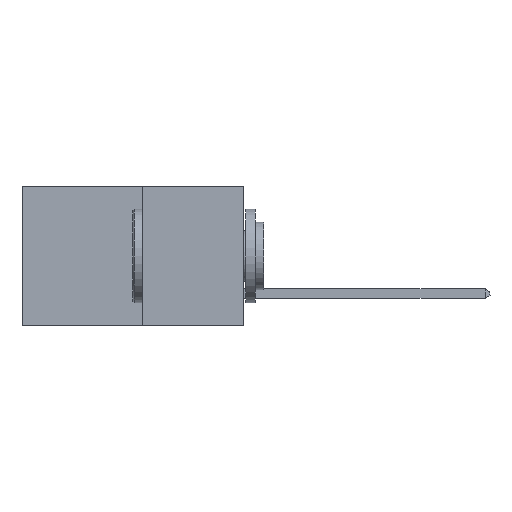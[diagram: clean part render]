
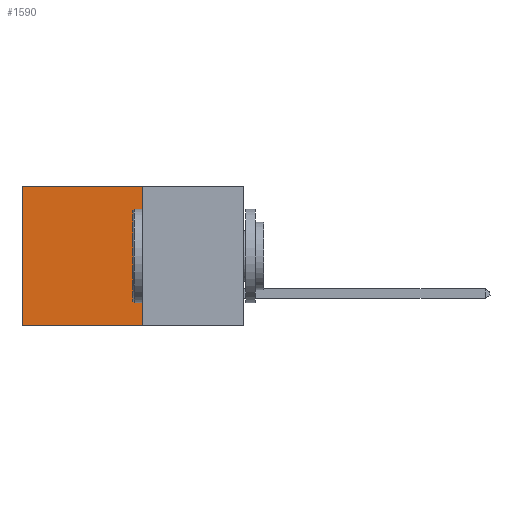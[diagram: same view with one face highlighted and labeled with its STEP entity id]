
A CAD part, left-side view. The second image highlights one B-rep face of the part: STEP entity #1590.
In plain terms, the highlighted planar face has unit normal (-1, 0, 0).
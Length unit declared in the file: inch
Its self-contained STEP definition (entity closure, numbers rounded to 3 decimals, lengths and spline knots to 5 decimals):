
#7 = VECTOR ( 'NONE', #5271, 39.37008 ) ;
#123 = VECTOR ( 'NONE', #1411, 39.37008 ) ;
#1164 = DIRECTION ( 'NONE',  ( 1., 0., 0. ) ) ;
#1337 = CARTESIAN_POINT ( 'NONE',  ( 0.277, 0.27, -0.37 ) ) ;
#1411 = DIRECTION ( 'NONE',  ( 0., 0., -1. ) ) ;
#1513 = CARTESIAN_POINT ( 'NONE',  ( 0.277, 0.59, -0.37 ) ) ;
#1590 = ADVANCED_FACE ( 'NONE', ( #9350 ), #10521, .F. ) ;
#2005 = VECTOR ( 'NONE', #6121, 39.37008 ) ;
#2497 = LINE ( 'NONE', #3972, #2005 ) ;
#2735 = EDGE_CURVE ( 'NONE', #3158, #8025, #2497, .T. ) ;
#2864 = CARTESIAN_POINT ( 'NONE',  ( 0.277, 0.59, -0.37 ) ) ;
#2947 = DIRECTION ( 'NONE',  ( 0., 0., -1. ) ) ;
#3130 = DIRECTION ( 'NONE',  ( 0., 0., -1. ) ) ;
#3158 = VERTEX_POINT ( 'NONE', #1337 ) ;
#3329 = CARTESIAN_POINT ( 'NONE',  ( 0.277, 0.27, -0.37 ) ) ;
#3543 = CARTESIAN_POINT ( 'NONE',  ( 0.277, 0.59, 0. ) ) ;
#3852 = CARTESIAN_POINT ( 'NONE',  ( 0.277, 0.27, -0.37 ) ) ;
#3972 = CARTESIAN_POINT ( 'NONE',  ( 0.277, 0.27, -0.37 ) ) ;
#4032 = EDGE_LOOP ( 'NONE', ( #5303, #7614, #10034, #7896 ) ) ;
#4145 = VERTEX_POINT ( 'NONE', #5506 ) ;
#4331 = VECTOR ( 'NONE', #3130, 39.37008 ) ;
#4714 = AXIS2_PLACEMENT_3D ( 'NONE', #3852, #1164, #2947 ) ;
#5271 = DIRECTION ( 'NONE',  ( 0., 1., 0. ) ) ;
#5303 = ORIENTED_EDGE ( 'NONE', *, *, #6540, .T. ) ;
#5506 = CARTESIAN_POINT ( 'NONE',  ( 0.277, 0.27, 0. ) ) ;
#5537 = VERTEX_POINT ( 'NONE', #3543 ) ;
#6121 = DIRECTION ( 'NONE',  ( 0., 1., 0. ) ) ;
#6396 = EDGE_CURVE ( 'NONE', #4145, #3158, #11365, .T. ) ;
#6540 = EDGE_CURVE ( 'NONE', #5537, #8025, #7324, .T. ) ;
#7324 = LINE ( 'NONE', #1513, #123 ) ;
#7614 = ORIENTED_EDGE ( 'NONE', *, *, #2735, .F. ) ;
#7896 = ORIENTED_EDGE ( 'NONE', *, *, #10696, .T. ) ;
#8025 = VERTEX_POINT ( 'NONE', #2864 ) ;
#9350 = FACE_OUTER_BOUND ( 'NONE', #4032, .T. ) ;
#9662 = CARTESIAN_POINT ( 'NONE',  ( 0.277, 0.27, 0. ) ) ;
#10034 = ORIENTED_EDGE ( 'NONE', *, *, #6396, .F. ) ;
#10521 = PLANE ( 'NONE',  #4714 ) ;
#10696 = EDGE_CURVE ( 'NONE', #4145, #5537, #11397, .T. ) ;
#11365 = LINE ( 'NONE', #3329, #4331 ) ;
#11397 = LINE ( 'NONE', #9662, #7 ) ;
